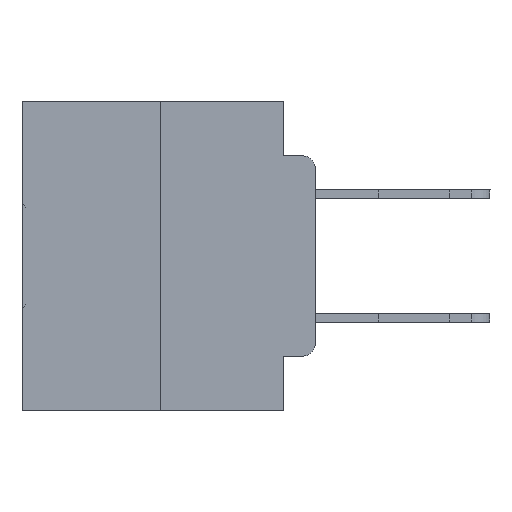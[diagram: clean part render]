
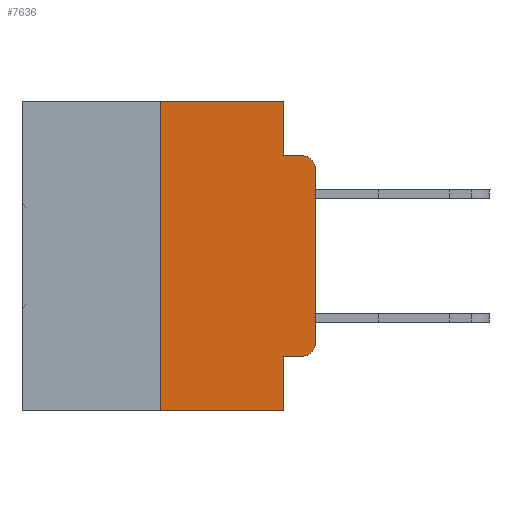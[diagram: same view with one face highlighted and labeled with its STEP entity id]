
A CAD part, left-side view. The second image highlights one B-rep face of the part: STEP entity #7636.
In plain terms, the highlighted planar face has unit normal (-1, 0, 0).
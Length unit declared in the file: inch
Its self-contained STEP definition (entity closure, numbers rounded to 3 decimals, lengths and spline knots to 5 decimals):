
#616 = AXIS2_PLACEMENT_3D ( 'NONE', #26679, #1431, #1288 ) ;
#670 = CARTESIAN_POINT ( 'NONE',  ( 0., 0.473, 0. ) ) ;
#1288 = DIRECTION ( 'NONE',  ( 0., 0., -1. ) ) ;
#1322 = CIRCLE ( 'NONE', #5499, 0.02 ) ;
#1431 = DIRECTION ( 'NONE',  ( -1., 0., 0. ) ) ;
#1729 = ORIENTED_EDGE ( 'NONE', *, *, #5639, .F. ) ;
#2196 = ORIENTED_EDGE ( 'NONE', *, *, #21357, .F. ) ;
#2288 = FACE_OUTER_BOUND ( 'NONE', #32254, .T. ) ;
#2444 = DIRECTION ( 'NONE',  ( 0., 0., -1. ) ) ;
#2547 = DIRECTION ( 'NONE',  ( 0., -1., 0. ) ) ;
#2644 = LINE ( 'NONE', #15269, #20866 ) ;
#2785 = VERTEX_POINT ( 'NONE', #10264 ) ;
#2901 = EDGE_CURVE ( 'NONE', #30063, #2785, #10103, .T. ) ;
#3419 = CARTESIAN_POINT ( 'NONE',  ( 0., 0.25, -0.5 ) ) ;
#3459 = LINE ( 'NONE', #670, #23636 ) ;
#3487 = ORIENTED_EDGE ( 'NONE', *, *, #19578, .T. ) ;
#3594 = LINE ( 'NONE', #11299, #29367 ) ;
#4049 = CARTESIAN_POINT ( 'NONE',  ( 0., 0.02, -0.4115 ) ) ;
#4065 = VERTEX_POINT ( 'NONE', #28172 ) ;
#4244 = VERTEX_POINT ( 'NONE', #3419 ) ;
#4652 = EDGE_CURVE ( 'NONE', #23637, #30063, #24469, .T. ) ;
#4913 = CARTESIAN_POINT ( 'NONE',  ( 0., 0.473, 0. ) ) ;
#5032 = EDGE_CURVE ( 'NONE', #26740, #23637, #3459, .T. ) ;
#5499 = AXIS2_PLACEMENT_3D ( 'NONE', #9771, #21900, #16999 ) ;
#5639 = EDGE_CURVE ( 'NONE', #4244, #26740, #27323, .T. ) ;
#6090 = DIRECTION ( 'NONE',  ( 0., -1., 0. ) ) ;
#6611 = DIRECTION ( 'NONE',  ( 0., 0., -1. ) ) ;
#7160 = VERTEX_POINT ( 'NONE', #12806 ) ;
#7223 = VERTEX_POINT ( 'NONE', #25599 ) ;
#7636 = ADVANCED_FACE ( 'NONE', ( #2288 ), #12286, .F. ) ;
#7641 = CARTESIAN_POINT ( 'NONE',  ( 0., 0.25, 0. ) ) ;
#7825 = CARTESIAN_POINT ( 'NONE',  ( 0., 0.051, -0.4115 ) ) ;
#9771 = CARTESIAN_POINT ( 'NONE',  ( 0., 0.02, -0.3915 ) ) ;
#10103 = LINE ( 'NONE', #10410, #29319 ) ;
#10264 = CARTESIAN_POINT ( 'NONE',  ( 0., 0.02, -0.0885 ) ) ;
#10410 = CARTESIAN_POINT ( 'NONE',  ( 0., 0.051, -0.0885 ) ) ;
#11299 = CARTESIAN_POINT ( 'NONE',  ( 0., 0., 0. ) ) ;
#12286 = PLANE ( 'NONE',  #24135 ) ;
#12461 = ORIENTED_EDGE ( 'NONE', *, *, #27470, .T. ) ;
#12806 = CARTESIAN_POINT ( 'NONE',  ( 0., 0.051, -0.5 ) ) ;
#13902 = EDGE_CURVE ( 'NONE', #4244, #7160, #2644, .T. ) ;
#14337 = CARTESIAN_POINT ( 'NONE',  ( 0., 0.051, -0.0885 ) ) ;
#14463 = EDGE_CURVE ( 'NONE', #17978, #7223, #3594, .T. ) ;
#14627 = VECTOR ( 'NONE', #22596, 39.37008 ) ;
#14687 = VECTOR ( 'NONE', #6611, 39.37008 ) ;
#14770 = VECTOR ( 'NONE', #23892, 39.37008 ) ;
#14909 = DIRECTION ( 'NONE',  ( 1., 0., 0. ) ) ;
#15269 = CARTESIAN_POINT ( 'NONE',  ( 0., 0.473, -0.5 ) ) ;
#16549 = DIRECTION ( 'NONE',  ( 0., 0., 1. ) ) ;
#16999 = DIRECTION ( 'NONE',  ( 0., 0., -1. ) ) ;
#17978 = VERTEX_POINT ( 'NONE', #26081 ) ;
#18480 = VERTEX_POINT ( 'NONE', #4049 ) ;
#18544 = VECTOR ( 'NONE', #19303, 39.37008 ) ;
#19303 = DIRECTION ( 'NONE',  ( 0., 0., 1. ) ) ;
#19373 = CARTESIAN_POINT ( 'NONE',  ( 0., 0.051, 0. ) ) ;
#19474 = ORIENTED_EDGE ( 'NONE', *, *, #4652, .F. ) ;
#19578 = EDGE_CURVE ( 'NONE', #7223, #2785, #24187, .T. ) ;
#19896 = ORIENTED_EDGE ( 'NONE', *, *, #14463, .T. ) ;
#20845 = DIRECTION ( 'NONE',  ( 0., -1., 0. ) ) ;
#20866 = VECTOR ( 'NONE', #20845, 39.37008 ) ;
#21357 = EDGE_CURVE ( 'NONE', #4065, #7160, #26512, .T. ) ;
#21900 = DIRECTION ( 'NONE',  ( -1., 0., 0. ) ) ;
#22596 = DIRECTION ( 'NONE',  ( 0., -1., 0. ) ) ;
#23447 = ORIENTED_EDGE ( 'NONE', *, *, #13902, .T. ) ;
#23636 = VECTOR ( 'NONE', #6090, 39.37008 ) ;
#23637 = VERTEX_POINT ( 'NONE', #30654 ) ;
#23892 = DIRECTION ( 'NONE',  ( 0., 0., -1. ) ) ;
#24034 = ORIENTED_EDGE ( 'NONE', *, *, #26702, .T. ) ;
#24135 = AXIS2_PLACEMENT_3D ( 'NONE', #4913, #14909, #2444 ) ;
#24187 = CIRCLE ( 'NONE', #616, 0.02 ) ;
#24469 = LINE ( 'NONE', #19373, #14687 ) ;
#25599 = CARTESIAN_POINT ( 'NONE',  ( 0., 0., -0.1085 ) ) ;
#26081 = CARTESIAN_POINT ( 'NONE',  ( 0., 0., -0.3915 ) ) ;
#26512 = LINE ( 'NONE', #31264, #14770 ) ;
#26679 = CARTESIAN_POINT ( 'NONE',  ( 0., 0.02, -0.1085 ) ) ;
#26702 = EDGE_CURVE ( 'NONE', #18480, #17978, #1322, .T. ) ;
#26740 = VERTEX_POINT ( 'NONE', #7641 ) ;
#27323 = LINE ( 'NONE', #29490, #18544 ) ;
#27470 = EDGE_CURVE ( 'NONE', #4065, #18480, #27526, .T. ) ;
#27526 = LINE ( 'NONE', #7825, #14627 ) ;
#28172 = CARTESIAN_POINT ( 'NONE',  ( 0., 0.051, -0.4115 ) ) ;
#28359 = ORIENTED_EDGE ( 'NONE', *, *, #2901, .F. ) ;
#29319 = VECTOR ( 'NONE', #2547, 39.37008 ) ;
#29367 = VECTOR ( 'NONE', #16549, 39.37008 ) ;
#29490 = CARTESIAN_POINT ( 'NONE',  ( 0., 0.25, 0. ) ) ;
#30037 = ORIENTED_EDGE ( 'NONE', *, *, #5032, .F. ) ;
#30063 = VERTEX_POINT ( 'NONE', #14337 ) ;
#30654 = CARTESIAN_POINT ( 'NONE',  ( 0., 0.051, 0. ) ) ;
#31264 = CARTESIAN_POINT ( 'NONE',  ( 0., 0.051, 0. ) ) ;
#32254 = EDGE_LOOP ( 'NONE', ( #19896, #3487, #28359, #19474, #30037, #1729, #23447, #2196, #12461, #24034 ) ) ;
